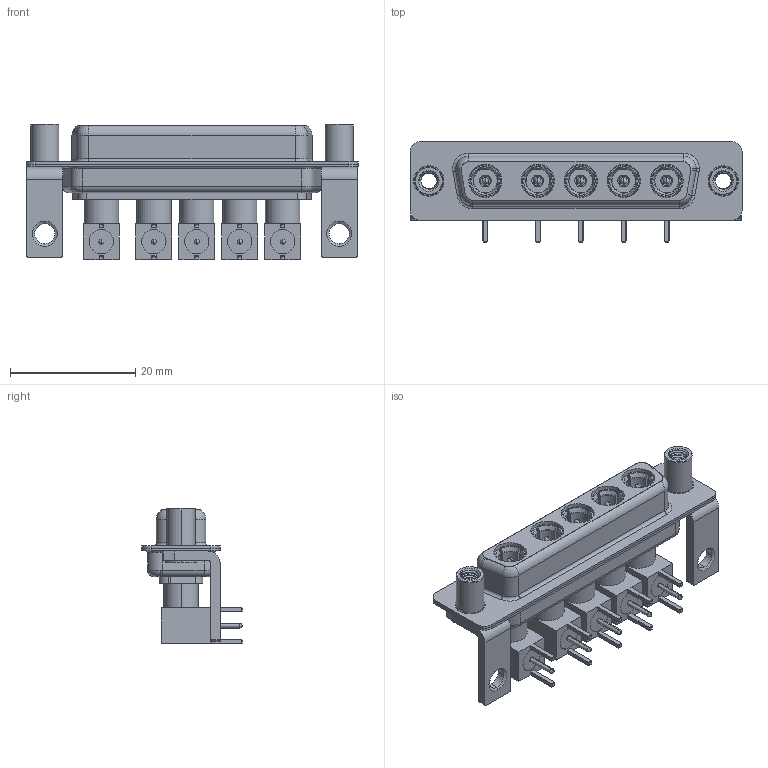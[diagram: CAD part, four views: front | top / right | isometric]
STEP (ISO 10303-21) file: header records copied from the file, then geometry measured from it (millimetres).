
FILE_DESCRIPTION (( 'STEP AP203' ), '1' );
FILE_NAME ('630-5W5-640-7TE.STEP', '2022-06-01T02:04:48', ( '' ), ( '' ), 'SwSTEP 2.0', 'SolidWorks 2020', '' );
FILE_SCHEMA (( 'CONFIG_CONTROL_DESIGN' ));
Length unit declared in the file: millimetre
Products named in the file (17): 630Combo Stabilizer Bracket; 630Combo Shell Rear_25 Contacts; Co-Ax Plug Assy_RA; Locking Collar; Insulator RA Pin; Co-Ax Plug_RA PC Tail; Insulator Pin_Straight PC Tail; 630-5W5-640-7TE; 630Combo Shell Front_25 Contacts; Pin_RA; 630Combo Housing_5W5; 630Combo Threaded Standoff_D; RA Back Shell
Assembly tree (42 placements, depth 3):
  630-5W5-640-7TE
    630Combo Housing_5W5
    630Combo Shell Front_25 Contacts
    630Combo Shell Rear_25 Contacts
    630Combo Stabilizer Bracket  x2
    630Combo Threaded Standoff_D  x2
    Co-Ax Plug Assy_RA
      Co-Ax Plug_RA PC Tail
      Insulator Pin_Straight PC Tail
      Pin_RA
      Locking Collar
      RA Back Shell
      Insulator RA Pin
    Co-Ax Plug Assy_RA
      Co-Ax Plug_RA PC Tail
      Insulator Pin_Straight PC Tail
      Pin_RA
      Locking Collar
      RA Back Shell
      Insulator RA Pin
    Co-Ax Plug Assy_RA
      Co-Ax Plug_RA PC Tail
      Insulator Pin_Straight PC Tail
      Pin_RA
      Locking Collar
      RA Back Shell
      Insulator RA Pin
    Co-Ax Plug Assy_RA
      Co-Ax Plug_RA PC Tail
      Insulator Pin_Straight PC Tail
      Pin_RA
      Locking Collar
      RA Back Shell
      Insulator RA Pin
    Co-Ax Plug Assy_RA
      Co-Ax Plug_RA PC Tail
      Insulator Pin_Straight PC Tail
      Pin_RA
      Locking Collar
      RA Back Shell
      Insulator RA Pin
Bounding box: 53.05 x 16 x 21.61 mm (x, y, z)
Volume: 5236.3 mm3; surface area: 12719.5 mm2
Topology: 37 solids, 37 shells, 1217 faces, 2960 edges, 1860 vertices
Faces by surface type: cylinder 534, plane 424, cone 141, torus 87, sphere 20, bspline 11
Entity records: 19352 total; most frequent: CARTESIAN_POINT 5213, DIRECTION 2606, ORIENTED_EDGE 2352, EDGE_CURVE 1176, AXIS2_PLACEMENT_3D 1047, VERTEX_POINT 745, EDGE_LOOP 549, CIRCLE 518
